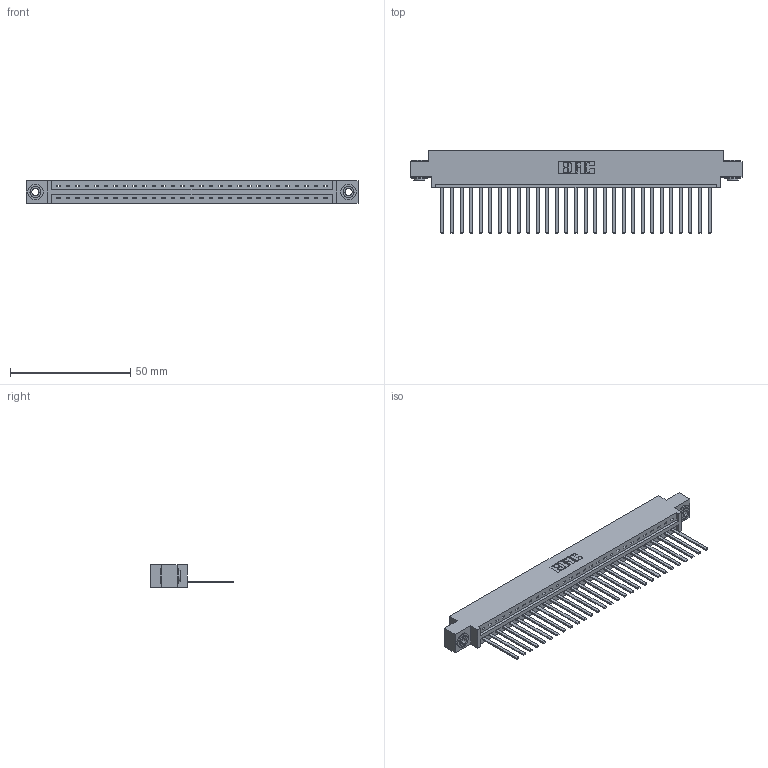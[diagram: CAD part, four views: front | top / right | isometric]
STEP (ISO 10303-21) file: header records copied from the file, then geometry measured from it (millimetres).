
FILE_DESCRIPTION (( 'STEP AP203' ), '1' );
FILE_NAME ('387-029-544-603.STEP', '2018-09-17T02:53:08', ( '' ), ( '' ), 'SwSTEP 2.0', 'SolidWorks 2016', '' );
FILE_SCHEMA (( 'CONFIG_CONTROL_DESIGN' ));
Length unit declared in the file: inch
Products named in the file (4): 345-292-001_345-293-144; 345-250-002_345-250-002-102; 387-029-544-603; 337 Part_0.170 Offset - 0.156 Dia-TH
Assembly tree (32 placements, depth 2):
  387-029-544-603
    337 Part_0.170 Offset - 0.156 Dia-TH
    345-292-001_345-293-144  x29
    345-250-002_345-250-002-102  x2
Bounding box: 137.92 x 34.3 x 9.4 mm (x, y, z)
Volume: 14409.7 mm3; surface area: 16252.1 mm2
Topology: 32 solids, 32 shells, 1780 faces, 5329 edges, 3510 vertices
Faces by surface type: plane 1302, cylinder 470, cone 8
Entity records: 23836 total; most frequent: CARTESIAN_POINT 4128, ORIENTED_EDGE 4086, DIRECTION 3531, EDGE_CURVE 2043, LINE 1895, VECTOR 1895, VERTEX_POINT 1358, AXIS2_PLACEMENT_3D 818
